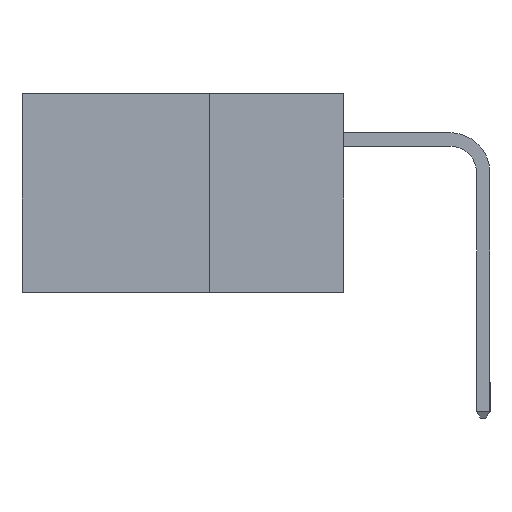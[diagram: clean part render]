
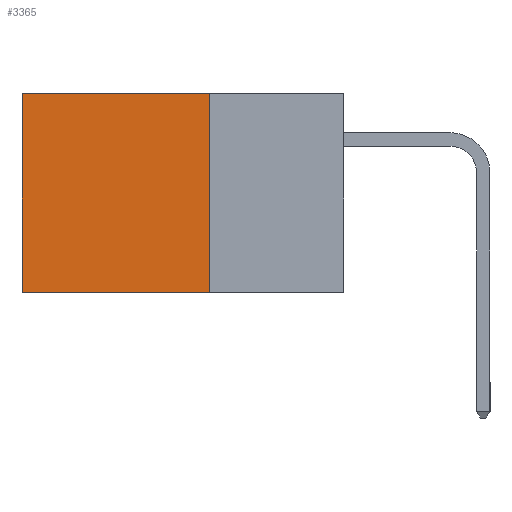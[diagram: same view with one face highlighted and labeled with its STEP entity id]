
A CAD part, left-side view. The second image highlights one B-rep face of the part: STEP entity #3365.
In plain terms, the highlighted planar face has unit normal (-1, 0, 0).
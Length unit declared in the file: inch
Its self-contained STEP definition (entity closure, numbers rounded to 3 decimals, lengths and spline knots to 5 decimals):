
#62 = AXIS2_PLACEMENT_3D ( 'NONE', #2178, #10276, #6825 ) ;
#180 = VECTOR ( 'NONE', #14533, 39.37008 ) ;
#427 = CARTESIAN_POINT ( 'NONE',  ( 0.298, 0.25, 0. ) ) ;
#1607 = LINE ( 'NONE', #4255, #180 ) ;
#1632 = DIRECTION ( 'NONE',  ( 0., 1., 0. ) ) ;
#1641 = ORIENTED_EDGE ( 'NONE', *, *, #5959, .T. ) ;
#2178 = CARTESIAN_POINT ( 'NONE',  ( 0.298, 0.25, 0. ) ) ;
#2729 = DIRECTION ( 'NONE',  ( 0., 0., -1. ) ) ;
#3032 = CARTESIAN_POINT ( 'NONE',  ( 0.298, 0.25, 0. ) ) ;
#3365 = ADVANCED_FACE ( 'NONE', ( #10483 ), #12513, .F. ) ;
#3428 = VECTOR ( 'NONE', #7868, 39.37008 ) ;
#3611 = VECTOR ( 'NONE', #1632, 39.37008 ) ;
#4255 = CARTESIAN_POINT ( 'NONE',  ( 0.298, 0.25, -0.37 ) ) ;
#4536 = ORIENTED_EDGE ( 'NONE', *, *, #7033, .T. ) ;
#4895 = EDGE_LOOP ( 'NONE', ( #4536, #12279, #7452, #1641 ) ) ;
#4929 = VERTEX_POINT ( 'NONE', #11783 ) ;
#5025 = EDGE_CURVE ( 'NONE', #8132, #4929, #5098, .T. ) ;
#5098 = LINE ( 'NONE', #8439, #9156 ) ;
#5558 = CARTESIAN_POINT ( 'NONE',  ( 0.298, 0.6, 0. ) ) ;
#5921 = CARTESIAN_POINT ( 'NONE',  ( 0.298, 0.6, 0. ) ) ;
#5959 = EDGE_CURVE ( 'NONE', #8132, #7876, #6491, .T. ) ;
#6036 = VERTEX_POINT ( 'NONE', #12649 ) ;
#6116 = LINE ( 'NONE', #5558, #3428 ) ;
#6491 = LINE ( 'NONE', #427, #3611 ) ;
#6825 = DIRECTION ( 'NONE',  ( 0., 0., -1. ) ) ;
#7033 = EDGE_CURVE ( 'NONE', #7876, #6036, #6116, .T. ) ;
#7452 = ORIENTED_EDGE ( 'NONE', *, *, #5025, .F. ) ;
#7868 = DIRECTION ( 'NONE',  ( 0., 0., -1. ) ) ;
#7876 = VERTEX_POINT ( 'NONE', #5921 ) ;
#8132 = VERTEX_POINT ( 'NONE', #3032 ) ;
#8439 = CARTESIAN_POINT ( 'NONE',  ( 0.298, 0.25, 0. ) ) ;
#9156 = VECTOR ( 'NONE', #2729, 39.37008 ) ;
#10276 = DIRECTION ( 'NONE',  ( 1., 0., 0. ) ) ;
#10483 = FACE_OUTER_BOUND ( 'NONE', #4895, .T. ) ;
#11783 = CARTESIAN_POINT ( 'NONE',  ( 0.298, 0.25, -0.37 ) ) ;
#12279 = ORIENTED_EDGE ( 'NONE', *, *, #12948, .F. ) ;
#12513 = PLANE ( 'NONE',  #62 ) ;
#12649 = CARTESIAN_POINT ( 'NONE',  ( 0.298, 0.6, -0.37 ) ) ;
#12948 = EDGE_CURVE ( 'NONE', #4929, #6036, #1607, .T. ) ;
#14533 = DIRECTION ( 'NONE',  ( 0., 1., 0. ) ) ;
